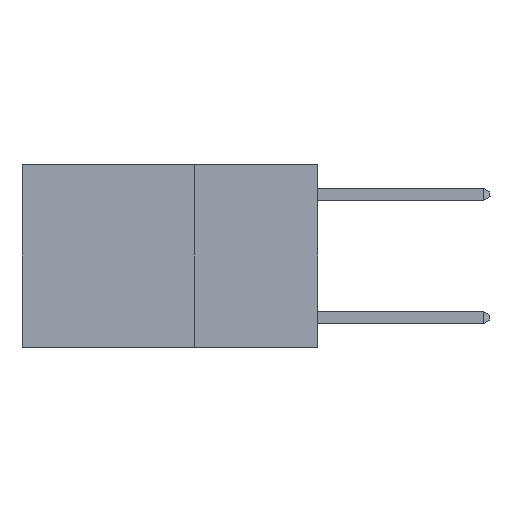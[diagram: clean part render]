
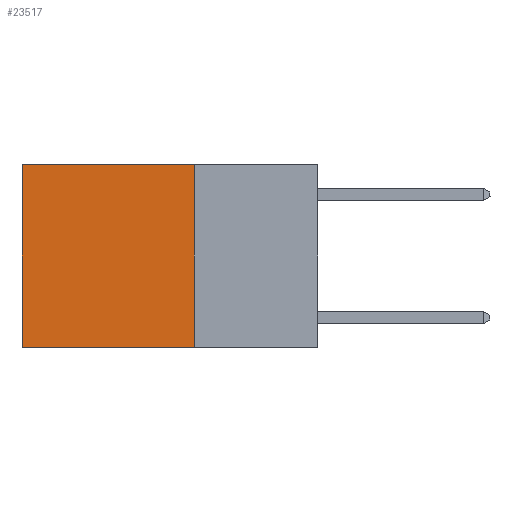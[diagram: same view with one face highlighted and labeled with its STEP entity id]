
A CAD part, left-side view. The second image highlights one B-rep face of the part: STEP entity #23517.
In plain terms, the highlighted planar face has unit normal (-1, 0, 0).
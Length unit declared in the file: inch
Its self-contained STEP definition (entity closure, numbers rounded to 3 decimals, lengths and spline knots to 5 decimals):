
#805 = CARTESIAN_POINT ( 'NONE',  ( 0.2625, 0.6, 0. ) ) ;
#958 = CARTESIAN_POINT ( 'NONE',  ( 0.2625, 0.6, -0.37 ) ) ;
#1214 = CARTESIAN_POINT ( 'NONE',  ( 0.2625, 0.25, 0. ) ) ;
#2371 = EDGE_CURVE ( 'NONE', #10089, #5623, #12008, .T. ) ;
#2417 = VECTOR ( 'NONE', #12137, 39.37008 ) ;
#2669 = EDGE_CURVE ( 'NONE', #5623, #8321, #6733, .T. ) ;
#3278 = VECTOR ( 'NONE', #21642, 39.37008 ) ;
#3515 = ORIENTED_EDGE ( 'NONE', *, *, #22196, .T. ) ;
#5623 = VERTEX_POINT ( 'NONE', #9517 ) ;
#6733 = LINE ( 'NONE', #11021, #10490 ) ;
#6976 = VECTOR ( 'NONE', #9289, 39.37008 ) ;
#7399 = FACE_OUTER_BOUND ( 'NONE', #20499, .T. ) ;
#8321 = VERTEX_POINT ( 'NONE', #958 ) ;
#9059 = CARTESIAN_POINT ( 'NONE',  ( 0.2625, 0.25, 0. ) ) ;
#9289 = DIRECTION ( 'NONE',  ( 0., 0., -1. ) ) ;
#9425 = LINE ( 'NONE', #805, #6976 ) ;
#9517 = CARTESIAN_POINT ( 'NONE',  ( 0.2625, 0.25, -0.37 ) ) ;
#10089 = VERTEX_POINT ( 'NONE', #1214 ) ;
#10420 = AXIS2_PLACEMENT_3D ( 'NONE', #9059, #20107, #17883 ) ;
#10490 = VECTOR ( 'NONE', #11292, 39.37008 ) ;
#11021 = CARTESIAN_POINT ( 'NONE',  ( 0.2625, 0.25, -0.37 ) ) ;
#11292 = DIRECTION ( 'NONE',  ( 0., 1., 0. ) ) ;
#12008 = LINE ( 'NONE', #22777, #2417 ) ;
#12137 = DIRECTION ( 'NONE',  ( 0., 0., -1. ) ) ;
#12300 = VERTEX_POINT ( 'NONE', #18998 ) ;
#15821 = PLANE ( 'NONE',  #10420 ) ;
#16322 = ORIENTED_EDGE ( 'NONE', *, *, #2669, .F. ) ;
#17883 = DIRECTION ( 'NONE',  ( 0., 0., -1. ) ) ;
#18998 = CARTESIAN_POINT ( 'NONE',  ( 0.2625, 0.6, 0. ) ) ;
#19686 = CARTESIAN_POINT ( 'NONE',  ( 0.2625, 0.25, 0. ) ) ;
#20107 = DIRECTION ( 'NONE',  ( 1., 0., 0. ) ) ;
#20499 = EDGE_LOOP ( 'NONE', ( #24278, #16322, #24257, #3515 ) ) ;
#21642 = DIRECTION ( 'NONE',  ( 0., 1., 0. ) ) ;
#21779 = LINE ( 'NONE', #19686, #3278 ) ;
#22196 = EDGE_CURVE ( 'NONE', #10089, #12300, #21779, .T. ) ;
#22777 = CARTESIAN_POINT ( 'NONE',  ( 0.2625, 0.25, 0. ) ) ;
#23517 = ADVANCED_FACE ( 'NONE', ( #7399 ), #15821, .F. ) ;
#24257 = ORIENTED_EDGE ( 'NONE', *, *, #2371, .F. ) ;
#24278 = ORIENTED_EDGE ( 'NONE', *, *, #25904, .T. ) ;
#25904 = EDGE_CURVE ( 'NONE', #12300, #8321, #9425, .T. ) ;
